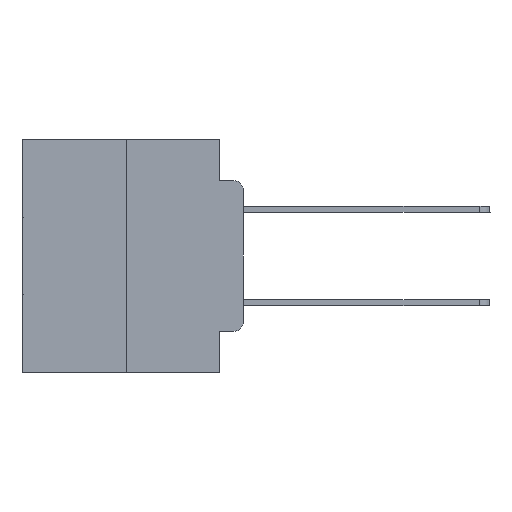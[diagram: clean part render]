
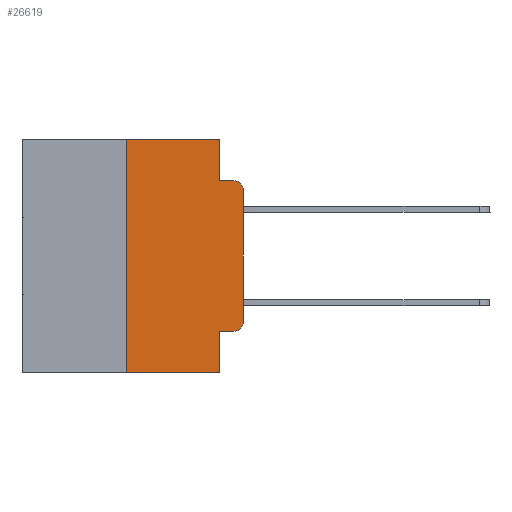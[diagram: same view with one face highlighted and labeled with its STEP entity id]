
A CAD part, left-side view. The second image highlights one B-rep face of the part: STEP entity #26619.
In plain terms, the highlighted planar face has unit normal (-1, 0, 0).
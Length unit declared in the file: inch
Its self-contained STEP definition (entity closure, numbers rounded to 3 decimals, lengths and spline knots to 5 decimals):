
#223 = CARTESIAN_POINT ( 'NONE',  ( 0., 0.473, 0. ) ) ;
#378 = DIRECTION ( 'NONE',  ( 0., -1., 0. ) ) ;
#455 = AXIS2_PLACEMENT_3D ( 'NONE', #19324, #14772, #27862 ) ;
#1127 = CARTESIAN_POINT ( 'NONE',  ( 0., 0.02, -0.1085 ) ) ;
#1170 = ORIENTED_EDGE ( 'NONE', *, *, #24215, .F. ) ;
#1229 = CARTESIAN_POINT ( 'NONE',  ( 0., 0.25, 0. ) ) ;
#1382 = CARTESIAN_POINT ( 'NONE',  ( 0., 0.051, -0.4115 ) ) ;
#1521 = DIRECTION ( 'NONE',  ( 0., 0., 1. ) ) ;
#2034 = EDGE_CURVE ( 'NONE', #24927, #21916, #23670, .T. ) ;
#2146 = DIRECTION ( 'NONE',  ( 1., 0., 0. ) ) ;
#2241 = EDGE_CURVE ( 'NONE', #17802, #22851, #8710, .T. ) ;
#2837 = EDGE_CURVE ( 'NONE', #3845, #20781, #12024, .T. ) ;
#2843 = VERTEX_POINT ( 'NONE', #25505 ) ;
#2890 = LINE ( 'NONE', #14591, #20533 ) ;
#2892 = CARTESIAN_POINT ( 'NONE',  ( 0., 0.051, 0. ) ) ;
#3309 = CARTESIAN_POINT ( 'NONE',  ( 0., 0.051, -0.5 ) ) ;
#3780 = CARTESIAN_POINT ( 'NONE',  ( 0., 0.051, -0.0885 ) ) ;
#3845 = VERTEX_POINT ( 'NONE', #3780 ) ;
#4205 = FACE_OUTER_BOUND ( 'NONE', #25301, .T. ) ;
#4648 = VECTOR ( 'NONE', #10067, 39.37008 ) ;
#4730 = DIRECTION ( 'NONE',  ( 0., 0., -1. ) ) ;
#4829 = VECTOR ( 'NONE', #13216, 39.37008 ) ;
#5614 = CARTESIAN_POINT ( 'NONE',  ( 0., 0.02, -0.0885 ) ) ;
#5628 = EDGE_CURVE ( 'NONE', #24274, #20781, #26164, .T. ) ;
#6117 = CARTESIAN_POINT ( 'NONE',  ( 0., 0.25, 0. ) ) ;
#6124 = DIRECTION ( 'NONE',  ( 0., -1., 0. ) ) ;
#6709 = LINE ( 'NONE', #1229, #8070 ) ;
#6983 = CARTESIAN_POINT ( 'NONE',  ( 0., 0.051, -0.4115 ) ) ;
#8070 = VECTOR ( 'NONE', #1521, 39.37008 ) ;
#8444 = CARTESIAN_POINT ( 'NONE',  ( 0., 0., -0.1085 ) ) ;
#8710 = LINE ( 'NONE', #17025, #26037 ) ;
#8771 = CARTESIAN_POINT ( 'NONE',  ( 0., 0.473, -0.5 ) ) ;
#9023 = VERTEX_POINT ( 'NONE', #14579 ) ;
#9288 = DIRECTION ( 'NONE',  ( -1., 0., 0. ) ) ;
#9370 = EDGE_CURVE ( 'NONE', #22851, #3845, #12165, .T. ) ;
#9565 = ORIENTED_EDGE ( 'NONE', *, *, #12973, .T. ) ;
#9898 = VECTOR ( 'NONE', #11752, 39.37008 ) ;
#10067 = DIRECTION ( 'NONE',  ( 0., 0., -1. ) ) ;
#10405 = ORIENTED_EDGE ( 'NONE', *, *, #2034, .F. ) ;
#11752 = DIRECTION ( 'NONE',  ( 0., -1., 0. ) ) ;
#12024 = LINE ( 'NONE', #23597, #19900 ) ;
#12165 = LINE ( 'NONE', #2892, #20349 ) ;
#12973 = EDGE_CURVE ( 'NONE', #9023, #24274, #2890, .T. ) ;
#13216 = DIRECTION ( 'NONE',  ( 0., -1., 0. ) ) ;
#13423 = ORIENTED_EDGE ( 'NONE', *, *, #27215, .T. ) ;
#13792 = ORIENTED_EDGE ( 'NONE', *, *, #22043, .T. ) ;
#14000 = LINE ( 'NONE', #6983, #9898 ) ;
#14003 = ORIENTED_EDGE ( 'NONE', *, *, #2241, .F. ) ;
#14495 = DIRECTION ( 'NONE',  ( 0., 0., 1. ) ) ;
#14579 = CARTESIAN_POINT ( 'NONE',  ( 0., 0., -0.3915 ) ) ;
#14591 = CARTESIAN_POINT ( 'NONE',  ( 0., 0., 0. ) ) ;
#14772 = DIRECTION ( 'NONE',  ( -1., 0., 0. ) ) ;
#14905 = VERTEX_POINT ( 'NONE', #25818 ) ;
#15769 = ORIENTED_EDGE ( 'NONE', *, *, #17947, .T. ) ;
#17025 = CARTESIAN_POINT ( 'NONE',  ( 0., 0.473, 0. ) ) ;
#17802 = VERTEX_POINT ( 'NONE', #6117 ) ;
#17947 = EDGE_CURVE ( 'NONE', #14905, #21916, #27233, .T. ) ;
#18154 = DIRECTION ( 'NONE',  ( 0., 0., -1. ) ) ;
#18741 = ORIENTED_EDGE ( 'NONE', *, *, #2837, .F. ) ;
#19324 = CARTESIAN_POINT ( 'NONE',  ( 0., 0.02, -0.3915 ) ) ;
#19900 = VECTOR ( 'NONE', #6124, 39.37008 ) ;
#20261 = PLANE ( 'NONE',  #27418 ) ;
#20349 = VECTOR ( 'NONE', #18154, 39.37008 ) ;
#20533 = VECTOR ( 'NONE', #14495, 39.37008 ) ;
#20781 = VERTEX_POINT ( 'NONE', #5614 ) ;
#20910 = CARTESIAN_POINT ( 'NONE',  ( 0., 0.051, 0. ) ) ;
#21374 = CIRCLE ( 'NONE', #455, 0.02 ) ;
#21916 = VERTEX_POINT ( 'NONE', #3309 ) ;
#22043 = EDGE_CURVE ( 'NONE', #2843, #9023, #21374, .T. ) ;
#22731 = ORIENTED_EDGE ( 'NONE', *, *, #9370, .F. ) ;
#22851 = VERTEX_POINT ( 'NONE', #27178 ) ;
#23263 = ORIENTED_EDGE ( 'NONE', *, *, #5628, .T. ) ;
#23597 = CARTESIAN_POINT ( 'NONE',  ( 0., 0.051, -0.0885 ) ) ;
#23670 = LINE ( 'NONE', #20910, #4648 ) ;
#24215 = EDGE_CURVE ( 'NONE', #14905, #17802, #6709, .T. ) ;
#24274 = VERTEX_POINT ( 'NONE', #8444 ) ;
#24927 = VERTEX_POINT ( 'NONE', #1382 ) ;
#25301 = EDGE_LOOP ( 'NONE', ( #9565, #23263, #18741, #22731, #14003, #1170, #15769, #10405, #13423, #13792 ) ) ;
#25505 = CARTESIAN_POINT ( 'NONE',  ( 0., 0.02, -0.4115 ) ) ;
#25818 = CARTESIAN_POINT ( 'NONE',  ( 0., 0.25, -0.5 ) ) ;
#26037 = VECTOR ( 'NONE', #378, 39.37008 ) ;
#26164 = CIRCLE ( 'NONE', #27092, 0.02 ) ;
#26619 = ADVANCED_FACE ( 'NONE', ( #4205 ), #20261, .F. ) ;
#27092 = AXIS2_PLACEMENT_3D ( 'NONE', #1127, #9288, #27309 ) ;
#27178 = CARTESIAN_POINT ( 'NONE',  ( 0., 0.051, 0. ) ) ;
#27215 = EDGE_CURVE ( 'NONE', #24927, #2843, #14000, .T. ) ;
#27233 = LINE ( 'NONE', #8771, #4829 ) ;
#27309 = DIRECTION ( 'NONE',  ( 0., 0., -1. ) ) ;
#27418 = AXIS2_PLACEMENT_3D ( 'NONE', #223, #2146, #4730 ) ;
#27862 = DIRECTION ( 'NONE',  ( 0., 0., -1. ) ) ;
